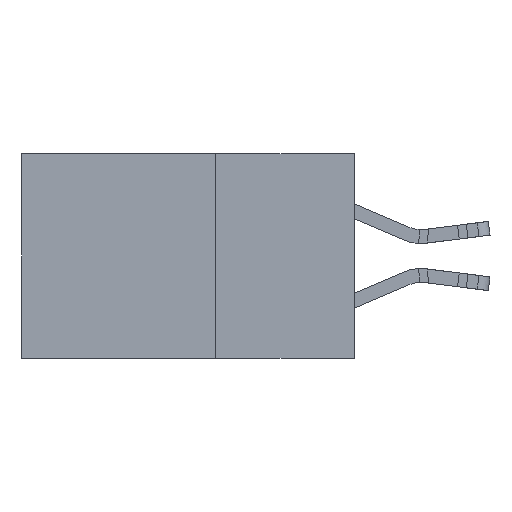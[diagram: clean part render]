
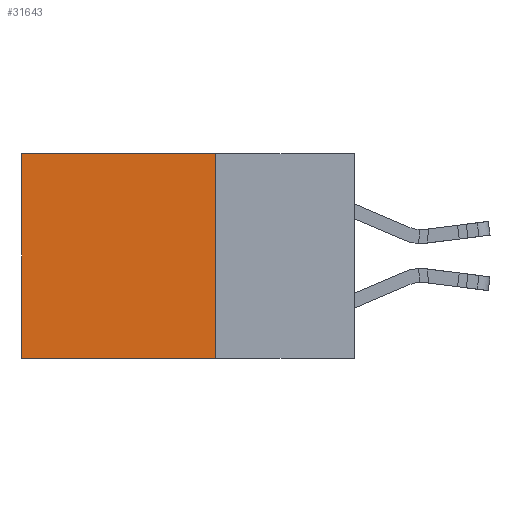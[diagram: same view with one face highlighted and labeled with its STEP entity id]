
A CAD part, left-side view. The second image highlights one B-rep face of the part: STEP entity #31643.
In plain terms, the highlighted planar face has unit normal (-1, 0, 0).
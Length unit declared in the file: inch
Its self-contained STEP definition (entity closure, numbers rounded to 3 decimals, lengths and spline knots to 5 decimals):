
#121 = VECTOR ( 'NONE', #27495, 39.37008 ) ;
#194 = DIRECTION ( 'NONE',  ( 0., 0., -1. ) ) ;
#221 = ORIENTED_EDGE ( 'NONE', *, *, #32617, .F. ) ;
#1122 = VECTOR ( 'NONE', #11632, 39.37008 ) ;
#2212 = CARTESIAN_POINT ( 'NONE',  ( 0.298, 0.25, 0. ) ) ;
#2781 = EDGE_LOOP ( 'NONE', ( #24116, #221, #4560, #30930 ) ) ;
#3649 = CARTESIAN_POINT ( 'NONE',  ( 0.298, 0.25, 0. ) ) ;
#4545 = FACE_OUTER_BOUND ( 'NONE', #2781, .T. ) ;
#4560 = ORIENTED_EDGE ( 'NONE', *, *, #5949, .F. ) ;
#5469 = DIRECTION ( 'NONE',  ( 0., 0., -1. ) ) ;
#5949 = EDGE_CURVE ( 'NONE', #21013, #17070, #10578, .T. ) ;
#6358 = CARTESIAN_POINT ( 'NONE',  ( 0.298, 0.25, 0. ) ) ;
#6955 = CARTESIAN_POINT ( 'NONE',  ( 0.298, 0.6, -0.37 ) ) ;
#7445 = DIRECTION ( 'NONE',  ( 0., 0., -1. ) ) ;
#8903 = AXIS2_PLACEMENT_3D ( 'NONE', #18617, #21254, #5469 ) ;
#10578 = LINE ( 'NONE', #2212, #29856 ) ;
#11161 = CARTESIAN_POINT ( 'NONE',  ( 0.298, 0.25, -0.37 ) ) ;
#11632 = DIRECTION ( 'NONE',  ( 0., 1., 0. ) ) ;
#13299 = PLANE ( 'NONE',  #8903 ) ;
#13313 = VECTOR ( 'NONE', #194, 39.37008 ) ;
#15181 = LINE ( 'NONE', #29973, #1122 ) ;
#16021 = CARTESIAN_POINT ( 'NONE',  ( 0.298, 0.6, 0. ) ) ;
#17070 = VERTEX_POINT ( 'NONE', #11161 ) ;
#17481 = EDGE_CURVE ( 'NONE', #22650, #17933, #33419, .T. ) ;
#17933 = VERTEX_POINT ( 'NONE', #6955 ) ;
#18617 = CARTESIAN_POINT ( 'NONE',  ( 0.298, 0.25, 0. ) ) ;
#21013 = VERTEX_POINT ( 'NONE', #3649 ) ;
#21240 = LINE ( 'NONE', #6358, #121 ) ;
#21254 = DIRECTION ( 'NONE',  ( 1., 0., 0. ) ) ;
#22650 = VERTEX_POINT ( 'NONE', #34011 ) ;
#23796 = EDGE_CURVE ( 'NONE', #21013, #22650, #21240, .T. ) ;
#24116 = ORIENTED_EDGE ( 'NONE', *, *, #17481, .T. ) ;
#27495 = DIRECTION ( 'NONE',  ( 0., 1., 0. ) ) ;
#29856 = VECTOR ( 'NONE', #7445, 39.37008 ) ;
#29973 = CARTESIAN_POINT ( 'NONE',  ( 0.298, 0.25, -0.37 ) ) ;
#30930 = ORIENTED_EDGE ( 'NONE', *, *, #23796, .T. ) ;
#31643 = ADVANCED_FACE ( 'NONE', ( #4545 ), #13299, .F. ) ;
#32617 = EDGE_CURVE ( 'NONE', #17070, #17933, #15181, .T. ) ;
#33419 = LINE ( 'NONE', #16021, #13313 ) ;
#34011 = CARTESIAN_POINT ( 'NONE',  ( 0.298, 0.6, 0. ) ) ;
